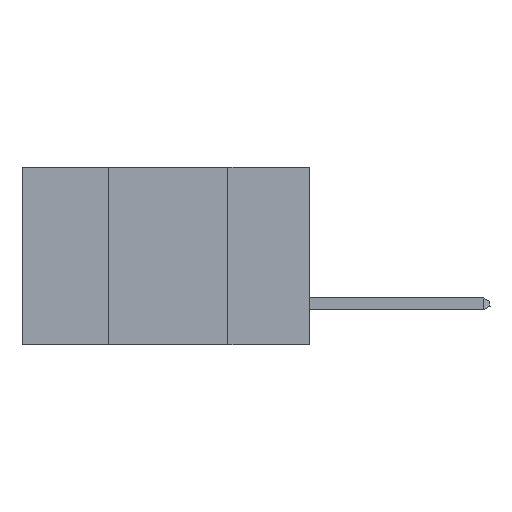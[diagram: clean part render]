
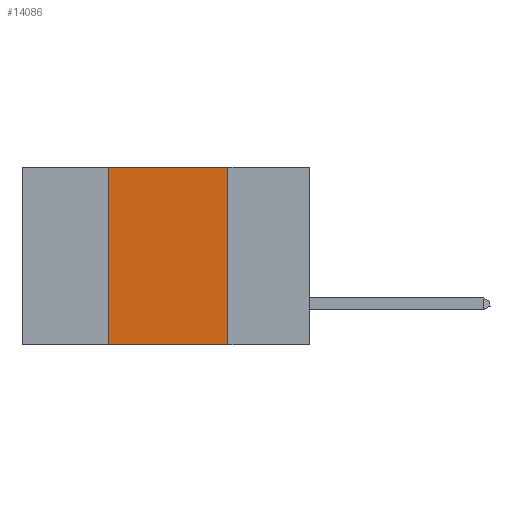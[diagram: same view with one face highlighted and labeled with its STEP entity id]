
A CAD part, left-side view. The second image highlights one B-rep face of the part: STEP entity #14086.
In plain terms, the highlighted planar face has unit normal (-1, 0, 0).
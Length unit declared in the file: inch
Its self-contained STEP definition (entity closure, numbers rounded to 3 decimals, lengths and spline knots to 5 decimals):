
#476 = LINE ( 'NONE', #10344, #4049 ) ;
#823 = CARTESIAN_POINT ( 'NONE',  ( 0., 0.17, -0.37 ) ) ;
#1216 = VECTOR ( 'NONE', #12922, 39.37008 ) ;
#2996 = DIRECTION ( 'NONE',  ( 0., 0., -1. ) ) ;
#3526 = ORIENTED_EDGE ( 'NONE', *, *, #7460, .T. ) ;
#3627 = EDGE_LOOP ( 'NONE', ( #9473, #11241, #5591, #3526 ) ) ;
#3740 = CARTESIAN_POINT ( 'NONE',  ( 0., 0.17, 0. ) ) ;
#4049 = VECTOR ( 'NONE', #13133, 39.37008 ) ;
#4187 = CARTESIAN_POINT ( 'NONE',  ( 0., 0.17, 0. ) ) ;
#4795 = LINE ( 'NONE', #10246, #1216 ) ;
#5591 = ORIENTED_EDGE ( 'NONE', *, *, #14332, .F. ) ;
#5594 = CARTESIAN_POINT ( 'NONE',  ( 0., 0.42, -0.37 ) ) ;
#7460 = EDGE_CURVE ( 'NONE', #12903, #12509, #476, .T. ) ;
#8801 = CARTESIAN_POINT ( 'NONE',  ( 0., 0.42, 0. ) ) ;
#9473 = ORIENTED_EDGE ( 'NONE', *, *, #11426, .F. ) ;
#9666 = AXIS2_PLACEMENT_3D ( 'NONE', #12662, #15391, #2996 ) ;
#9848 = VECTOR ( 'NONE', #15722, 39.37008 ) ;
#9930 = VECTOR ( 'NONE', #17390, 39.37008 ) ;
#10246 = CARTESIAN_POINT ( 'NONE',  ( 0., 0.6, 0. ) ) ;
#10344 = CARTESIAN_POINT ( 'NONE',  ( 0., 0.6, -0.37 ) ) ;
#11241 = ORIENTED_EDGE ( 'NONE', *, *, #13696, .F. ) ;
#11426 = EDGE_CURVE ( 'NONE', #12267, #12509, #14373, .T. ) ;
#11618 = CARTESIAN_POINT ( 'NONE',  ( 0., 0.42, 0. ) ) ;
#12267 = VERTEX_POINT ( 'NONE', #4187 ) ;
#12509 = VERTEX_POINT ( 'NONE', #823 ) ;
#12608 = PLANE ( 'NONE',  #9666 ) ;
#12662 = CARTESIAN_POINT ( 'NONE',  ( 0., 0.6, 0. ) ) ;
#12903 = VERTEX_POINT ( 'NONE', #5594 ) ;
#12922 = DIRECTION ( 'NONE',  ( 0., -1., 0. ) ) ;
#13133 = DIRECTION ( 'NONE',  ( 0., -1., 0. ) ) ;
#13696 = EDGE_CURVE ( 'NONE', #15631, #12267, #4795, .T. ) ;
#14086 = ADVANCED_FACE ( 'NONE', ( #16631 ), #12608, .F. ) ;
#14332 = EDGE_CURVE ( 'NONE', #12903, #15631, #17046, .T. ) ;
#14373 = LINE ( 'NONE', #3740, #9930 ) ;
#15391 = DIRECTION ( 'NONE',  ( 1., 0., 0. ) ) ;
#15631 = VERTEX_POINT ( 'NONE', #11618 ) ;
#15722 = DIRECTION ( 'NONE',  ( 0., 0., 1. ) ) ;
#16631 = FACE_OUTER_BOUND ( 'NONE', #3627, .T. ) ;
#17046 = LINE ( 'NONE', #8801, #9848 ) ;
#17390 = DIRECTION ( 'NONE',  ( 0., 0., -1. ) ) ;
